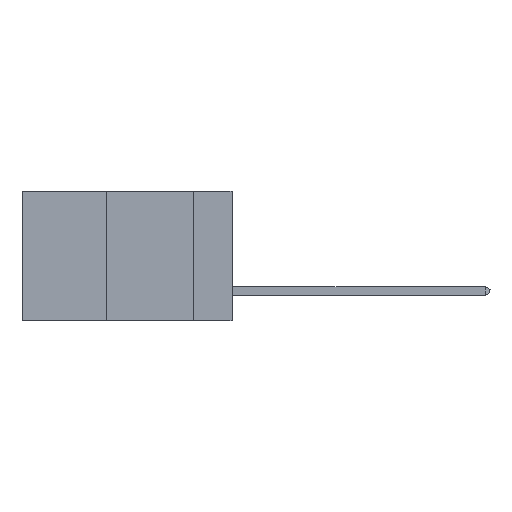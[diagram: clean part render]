
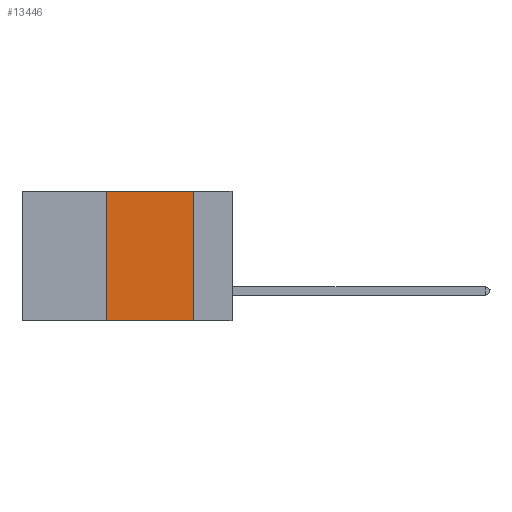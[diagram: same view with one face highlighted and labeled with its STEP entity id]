
A CAD part, left-side view. The second image highlights one B-rep face of the part: STEP entity #13446.
In plain terms, the highlighted planar face has unit normal (-1, 0, 0).
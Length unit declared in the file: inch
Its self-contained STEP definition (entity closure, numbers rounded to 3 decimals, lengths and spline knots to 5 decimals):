
#965 = EDGE_CURVE ( 'NONE', #18611, #1505, #18266, .T. ) ;
#1505 = VERTEX_POINT ( 'NONE', #15979 ) ;
#1813 = LINE ( 'NONE', #19301, #17324 ) ;
#2055 = CARTESIAN_POINT ( 'NONE',  ( 0., 0.11, -0.37 ) ) ;
#2479 = FACE_OUTER_BOUND ( 'NONE', #2832, .T. ) ;
#2643 = CARTESIAN_POINT ( 'NONE',  ( 0., 0.6, 0. ) ) ;
#2719 = LINE ( 'NONE', #21065, #12436 ) ;
#2777 = CARTESIAN_POINT ( 'NONE',  ( 0., 0.11, 0. ) ) ;
#2832 = EDGE_LOOP ( 'NONE', ( #19155, #12545, #4209, #6367 ) ) ;
#3082 = DIRECTION ( 'NONE',  ( 0., 0., 1. ) ) ;
#3223 = CARTESIAN_POINT ( 'NONE',  ( 0., 0.36, 0. ) ) ;
#4209 = ORIENTED_EDGE ( 'NONE', *, *, #965, .F. ) ;
#4573 = DIRECTION ( 'NONE',  ( 1., 0., 0. ) ) ;
#6042 = EDGE_CURVE ( 'NONE', #18611, #20926, #2719, .T. ) ;
#6367 = ORIENTED_EDGE ( 'NONE', *, *, #6042, .T. ) ;
#8534 = LINE ( 'NONE', #12997, #11566 ) ;
#11566 = VECTOR ( 'NONE', #13135, 39.37008 ) ;
#12436 = VECTOR ( 'NONE', #13036, 39.37008 ) ;
#12545 = ORIENTED_EDGE ( 'NONE', *, *, #17813, .F. ) ;
#12997 = CARTESIAN_POINT ( 'NONE',  ( 0., 0.11, 0. ) ) ;
#13036 = DIRECTION ( 'NONE',  ( 0., -1., 0. ) ) ;
#13135 = DIRECTION ( 'NONE',  ( 0., 0., -1. ) ) ;
#13446 = ADVANCED_FACE ( 'NONE', ( #2479 ), #15882, .F. ) ;
#15882 = PLANE ( 'NONE',  #19222 ) ;
#15979 = CARTESIAN_POINT ( 'NONE',  ( 0., 0.36, 0. ) ) ;
#16243 = EDGE_CURVE ( 'NONE', #18426, #20926, #8534, .T. ) ;
#16412 = CARTESIAN_POINT ( 'NONE',  ( 0., 0.36, -0.37 ) ) ;
#16538 = DIRECTION ( 'NONE',  ( 0., -1., 0. ) ) ;
#16752 = VECTOR ( 'NONE', #3082, 39.37008 ) ;
#17324 = VECTOR ( 'NONE', #16538, 39.37008 ) ;
#17813 = EDGE_CURVE ( 'NONE', #1505, #18426, #1813, .T. ) ;
#18266 = LINE ( 'NONE', #3223, #16752 ) ;
#18426 = VERTEX_POINT ( 'NONE', #2777 ) ;
#18611 = VERTEX_POINT ( 'NONE', #16412 ) ;
#19155 = ORIENTED_EDGE ( 'NONE', *, *, #16243, .F. ) ;
#19222 = AXIS2_PLACEMENT_3D ( 'NONE', #2643, #4573, #20661 ) ;
#19301 = CARTESIAN_POINT ( 'NONE',  ( 0., 0.6, 0. ) ) ;
#20661 = DIRECTION ( 'NONE',  ( 0., 0., -1. ) ) ;
#20926 = VERTEX_POINT ( 'NONE', #2055 ) ;
#21065 = CARTESIAN_POINT ( 'NONE',  ( 0., 0.6, -0.37 ) ) ;
